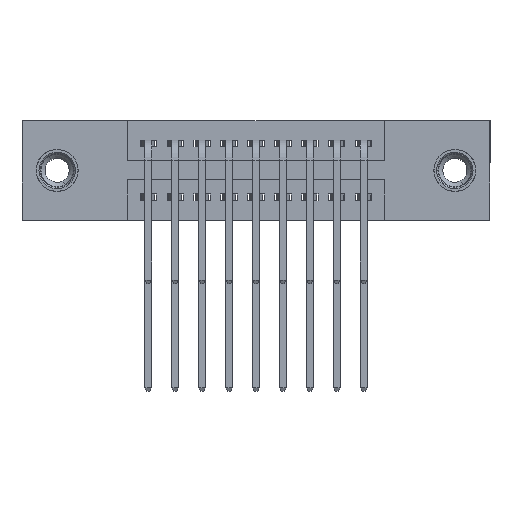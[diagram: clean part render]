
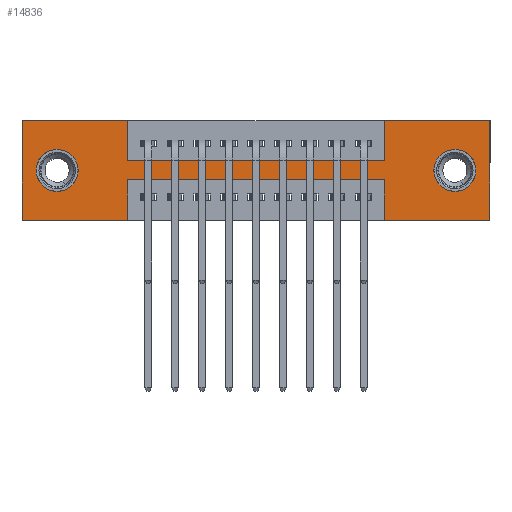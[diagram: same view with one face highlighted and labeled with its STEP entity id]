
A CAD part, front view. The second image highlights one B-rep face of the part: STEP entity #14836.
In plain terms, the highlighted planar face has unit normal (0, -1, 0).
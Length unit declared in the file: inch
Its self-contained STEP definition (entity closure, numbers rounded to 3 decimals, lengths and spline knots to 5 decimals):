
#61 = EDGE_CURVE ( 'NONE', #15282, #9262, #10169, .T. ) ;
#161 = VERTEX_POINT ( 'NONE', #11315 ) ;
#192 = ORIENTED_EDGE ( 'NONE', *, *, #61, .F. ) ;
#278 = ORIENTED_EDGE ( 'NONE', *, *, #15687, .F. ) ;
#427 = ORIENTED_EDGE ( 'NONE', *, *, #12250, .F. ) ;
#479 = CARTESIAN_POINT ( 'NONE',  ( 0.3925, 0., -0.22 ) ) ;
#609 = CARTESIAN_POINT ( 'NONE',  ( 0.3925, 0., -0.37 ) ) ;
#656 = EDGE_CURVE ( 'NONE', #5141, #161, #5679, .T. ) ;
#815 = DIRECTION ( 'NONE',  ( 0., 0., 1. ) ) ;
#869 = VERTEX_POINT ( 'NONE', #4306 ) ;
#957 = EDGE_CURVE ( 'NONE', #7728, #2960, #16734, .T. ) ;
#996 = VECTOR ( 'NONE', #1341, 39.37008 ) ;
#1199 = CARTESIAN_POINT ( 'NONE',  ( 0.13, 0., -0.185 ) ) ;
#1282 = AXIS2_PLACEMENT_3D ( 'NONE', #3367, #12825, #4727 ) ;
#1341 = DIRECTION ( 'NONE',  ( 1., 0., 0. ) ) ;
#1407 = CARTESIAN_POINT ( 'NONE',  ( 1.3425, 0., -0.22 ) ) ;
#1629 = LINE ( 'NONE', #13259, #16206 ) ;
#1631 = ORIENTED_EDGE ( 'NONE', *, *, #8756, .F. ) ;
#1717 = DIRECTION ( 'NONE',  ( 0., 1., 0. ) ) ;
#1734 = ORIENTED_EDGE ( 'NONE', *, *, #656, .F. ) ;
#1786 = DIRECTION ( 'NONE',  ( 0., 0., -1. ) ) ;
#1921 = VECTOR ( 'NONE', #10073, 39.37008 ) ;
#1924 = ORIENTED_EDGE ( 'NONE', *, *, #957, .T. ) ;
#1926 = DIRECTION ( 'NONE',  ( 0., 1., 0. ) ) ;
#1943 = CARTESIAN_POINT ( 'NONE',  ( 1.3425, 0., 0. ) ) ;
#2167 = CARTESIAN_POINT ( 'NONE',  ( 1.605, 0., -0.185 ) ) ;
#2340 = EDGE_CURVE ( 'NONE', #8487, #17359, #16062, .T. ) ;
#2385 = ORIENTED_EDGE ( 'NONE', *, *, #5630, .T. ) ;
#2733 = DIRECTION ( 'NONE',  ( 0., 0., 1. ) ) ;
#2915 = CARTESIAN_POINT ( 'NONE',  ( 1.735, 0., -0.37 ) ) ;
#2960 = VERTEX_POINT ( 'NONE', #8370 ) ;
#3034 = DIRECTION ( 'NONE',  ( -1., 0., 0. ) ) ;
#3084 = CARTESIAN_POINT ( 'NONE',  ( 0.3925, 0., -0.15 ) ) ;
#3100 = ORIENTED_EDGE ( 'NONE', *, *, #2340, .F. ) ;
#3121 = CARTESIAN_POINT ( 'NONE',  ( 0., 0., -0.37 ) ) ;
#3302 = ORIENTED_EDGE ( 'NONE', *, *, #14013, .F. ) ;
#3367 = CARTESIAN_POINT ( 'NONE',  ( 0.13, 0., -0.185 ) ) ;
#3494 = AXIS2_PLACEMENT_3D ( 'NONE', #2167, #1717, #1786 ) ;
#3567 = VERTEX_POINT ( 'NONE', #9475 ) ;
#3663 = CARTESIAN_POINT ( 'NONE',  ( 0.3925, 0., -0.22 ) ) ;
#3727 = ORIENTED_EDGE ( 'NONE', *, *, #15292, .F. ) ;
#3866 = VERTEX_POINT ( 'NONE', #8764 ) ;
#3926 = VECTOR ( 'NONE', #16613, 39.37008 ) ;
#4306 = CARTESIAN_POINT ( 'NONE',  ( 0.13, 0., -0.263 ) ) ;
#4727 = DIRECTION ( 'NONE',  ( 0., 0., 1. ) ) ;
#5071 = DIRECTION ( 'NONE',  ( 1., 0., 0. ) ) ;
#5141 = VERTEX_POINT ( 'NONE', #1943 ) ;
#5217 = CARTESIAN_POINT ( 'NONE',  ( 0., 0., 0. ) ) ;
#5245 = LINE ( 'NONE', #5836, #996 ) ;
#5411 = CARTESIAN_POINT ( 'NONE',  ( 0., 0., -0.37 ) ) ;
#5610 = LINE ( 'NONE', #11444, #1921 ) ;
#5630 = EDGE_CURVE ( 'NONE', #2960, #7728, #15322, .T. ) ;
#5679 = LINE ( 'NONE', #5217, #12478 ) ;
#5836 = CARTESIAN_POINT ( 'NONE',  ( 0., 0., 0. ) ) ;
#5917 = EDGE_LOOP ( 'NONE', ( #3302, #3727, #10946, #11374, #278, #1734, #8470, #1631, #3100, #8355, #427, #192 ) ) ;
#5920 = EDGE_CURVE ( 'NONE', #3567, #5141, #17647, .T. ) ;
#6036 = ORIENTED_EDGE ( 'NONE', *, *, #15534, .T. ) ;
#6177 = CARTESIAN_POINT ( 'NONE',  ( 0.3925, 0., -0.37 ) ) ;
#6532 = VECTOR ( 'NONE', #3034, 39.37008 ) ;
#6786 = VECTOR ( 'NONE', #16060, 39.37008 ) ;
#7728 = VERTEX_POINT ( 'NONE', #12122 ) ;
#7853 = VECTOR ( 'NONE', #12224, 39.37008 ) ;
#7902 = CARTESIAN_POINT ( 'NONE',  ( 1.3425, 0., 0. ) ) ;
#7938 = LINE ( 'NONE', #3663, #11564 ) ;
#8047 = PLANE ( 'NONE',  #15369 ) ;
#8355 = ORIENTED_EDGE ( 'NONE', *, *, #13856, .F. ) ;
#8370 = CARTESIAN_POINT ( 'NONE',  ( 1.605, 0., -0.263 ) ) ;
#8470 = ORIENTED_EDGE ( 'NONE', *, *, #5920, .F. ) ;
#8487 = VERTEX_POINT ( 'NONE', #13267 ) ;
#8546 = VERTEX_POINT ( 'NONE', #13386 ) ;
#8756 = EDGE_CURVE ( 'NONE', #17359, #3567, #11152, .T. ) ;
#8764 = CARTESIAN_POINT ( 'NONE',  ( 0., 0., 0. ) ) ;
#9262 = VERTEX_POINT ( 'NONE', #5411 ) ;
#9342 = VERTEX_POINT ( 'NONE', #1407 ) ;
#9349 = VERTEX_POINT ( 'NONE', #2915 ) ;
#9404 = DIRECTION ( 'NONE',  ( 0., 0., -1. ) ) ;
#9462 = VECTOR ( 'NONE', #15719, 39.37008 ) ;
#9475 = CARTESIAN_POINT ( 'NONE',  ( 1.3425, 0., -0.15 ) ) ;
#9617 = LINE ( 'NONE', #15299, #16447 ) ;
#10073 = DIRECTION ( 'NONE',  ( -1., 0., 0. ) ) ;
#10084 = ORIENTED_EDGE ( 'NONE', *, *, #13934, .T. ) ;
#10149 = CARTESIAN_POINT ( 'NONE',  ( 1.605, 0., -0.185 ) ) ;
#10169 = LINE ( 'NONE', #3121, #6532 ) ;
#10359 = EDGE_LOOP ( 'NONE', ( #1924, #2385 ) ) ;
#10861 = CARTESIAN_POINT ( 'NONE',  ( 0., 0., 0. ) ) ;
#10895 = DIRECTION ( 'NONE',  ( 0., 1., 0. ) ) ;
#10946 = ORIENTED_EDGE ( 'NONE', *, *, #11056, .F. ) ;
#11056 = EDGE_CURVE ( 'NONE', #15090, #9342, #1629, .T. ) ;
#11138 = CARTESIAN_POINT ( 'NONE',  ( 0.3925, 0., -0.15 ) ) ;
#11152 = LINE ( 'NONE', #11138, #3926 ) ;
#11211 = CARTESIAN_POINT ( 'NONE',  ( 1.3425, 0., -0.37 ) ) ;
#11315 = CARTESIAN_POINT ( 'NONE',  ( 1.735, 0., 0. ) ) ;
#11374 = ORIENTED_EDGE ( 'NONE', *, *, #15205, .F. ) ;
#11444 = CARTESIAN_POINT ( 'NONE',  ( 0., 0., -0.37 ) ) ;
#11482 = LINE ( 'NONE', #10861, #7853 ) ;
#11511 = DIRECTION ( 'NONE',  ( 0., 0., -1. ) ) ;
#11564 = VECTOR ( 'NONE', #11782, 39.37008 ) ;
#11782 = DIRECTION ( 'NONE',  ( -1., 0., 0. ) ) ;
#12006 = FACE_OUTER_BOUND ( 'NONE', #5917, .T. ) ;
#12041 = CARTESIAN_POINT ( 'NONE',  ( 0., 0., -0.37 ) ) ;
#12122 = CARTESIAN_POINT ( 'NONE',  ( 1.605, 0., -0.107 ) ) ;
#12224 = DIRECTION ( 'NONE',  ( 0., 0., 1. ) ) ;
#12250 = EDGE_CURVE ( 'NONE', #9262, #3866, #11482, .T. ) ;
#12433 = VECTOR ( 'NONE', #13302, 39.37008 ) ;
#12478 = VECTOR ( 'NONE', #5071, 39.37008 ) ;
#12647 = VERTEX_POINT ( 'NONE', #479 ) ;
#12825 = DIRECTION ( 'NONE',  ( 0., 1., 0. ) ) ;
#13079 = LINE ( 'NONE', #6177, #9462 ) ;
#13259 = CARTESIAN_POINT ( 'NONE',  ( 1.3425, 0., -0.37 ) ) ;
#13267 = CARTESIAN_POINT ( 'NONE',  ( 0.3925, 0., 0. ) ) ;
#13302 = DIRECTION ( 'NONE',  ( 0., 0., -1. ) ) ;
#13315 = CARTESIAN_POINT ( 'NONE',  ( 0.3925, 0., 0. ) ) ;
#13386 = CARTESIAN_POINT ( 'NONE',  ( 0.13, 0., -0.107 ) ) ;
#13856 = EDGE_CURVE ( 'NONE', #3866, #8487, #5245, .T. ) ;
#13934 = EDGE_CURVE ( 'NONE', #869, #8546, #14365, .T. ) ;
#14013 = EDGE_CURVE ( 'NONE', #12647, #15282, #13079, .T. ) ;
#14365 = CIRCLE ( 'NONE', #1282, 0.078 ) ;
#14665 = AXIS2_PLACEMENT_3D ( 'NONE', #1199, #10895, #2733 ) ;
#14770 = FACE_BOUND ( 'NONE', #10359, .T. ) ;
#14836 = ADVANCED_FACE ( 'NONE', ( #14770, #16061, #12006 ), #8047, .T. ) ;
#15090 = VERTEX_POINT ( 'NONE', #11211 ) ;
#15205 = EDGE_CURVE ( 'NONE', #9349, #15090, #5610, .T. ) ;
#15282 = VERTEX_POINT ( 'NONE', #609 ) ;
#15292 = EDGE_CURVE ( 'NONE', #9342, #12647, #7938, .T. ) ;
#15299 = CARTESIAN_POINT ( 'NONE',  ( 1.735, 0., 0. ) ) ;
#15322 = CIRCLE ( 'NONE', #17623, 0.078 ) ;
#15369 = AXIS2_PLACEMENT_3D ( 'NONE', #12041, #17563, #9404 ) ;
#15534 = EDGE_CURVE ( 'NONE', #8546, #869, #15828, .T. ) ;
#15687 = EDGE_CURVE ( 'NONE', #161, #9349, #9617, .T. ) ;
#15719 = DIRECTION ( 'NONE',  ( 0., 0., -1. ) ) ;
#15828 = CIRCLE ( 'NONE', #14665, 0.078 ) ;
#16060 = DIRECTION ( 'NONE',  ( 0., 0., 1. ) ) ;
#16061 = FACE_BOUND ( 'NONE', #17438, .T. ) ;
#16062 = LINE ( 'NONE', #13315, #12433 ) ;
#16206 = VECTOR ( 'NONE', #815, 39.37008 ) ;
#16447 = VECTOR ( 'NONE', #16650, 39.37008 ) ;
#16613 = DIRECTION ( 'NONE',  ( 1., 0., 0. ) ) ;
#16650 = DIRECTION ( 'NONE',  ( 0., 0., -1. ) ) ;
#16734 = CIRCLE ( 'NONE', #3494, 0.078 ) ;
#17359 = VERTEX_POINT ( 'NONE', #3084 ) ;
#17438 = EDGE_LOOP ( 'NONE', ( #6036, #10084 ) ) ;
#17563 = DIRECTION ( 'NONE',  ( 0., -1., 0. ) ) ;
#17623 = AXIS2_PLACEMENT_3D ( 'NONE', #10149, #1926, #11511 ) ;
#17647 = LINE ( 'NONE', #7902, #6786 ) ;
